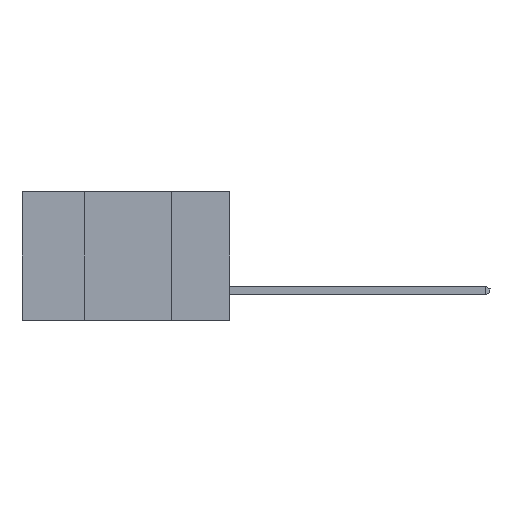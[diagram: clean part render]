
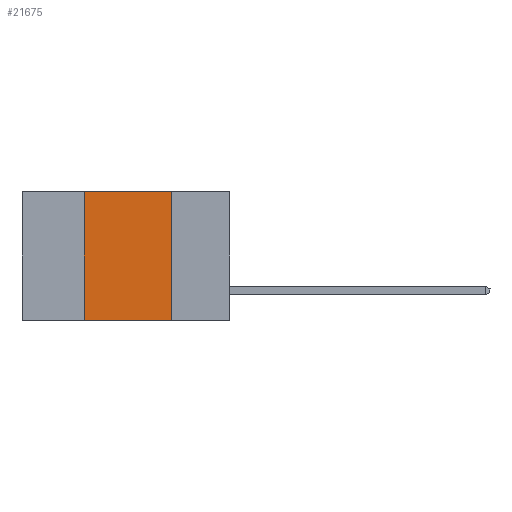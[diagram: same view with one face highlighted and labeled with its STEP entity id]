
A CAD part, left-side view. The second image highlights one B-rep face of the part: STEP entity #21675.
In plain terms, the highlighted planar face has unit normal (-1, 0, 0).
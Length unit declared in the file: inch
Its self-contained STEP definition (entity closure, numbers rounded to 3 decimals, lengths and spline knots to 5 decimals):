
#1277 = CARTESIAN_POINT ( 'NONE',  ( 0., 0.17, -0.37 ) ) ;
#1334 = CARTESIAN_POINT ( 'NONE',  ( 0., 0.6, 0. ) ) ;
#1555 = ORIENTED_EDGE ( 'NONE', *, *, #13676, .F. ) ;
#1757 = VECTOR ( 'NONE', #6043, 39.37008 ) ;
#1799 = DIRECTION ( 'NONE',  ( 1., 0., 0. ) ) ;
#2335 = CARTESIAN_POINT ( 'NONE',  ( 0., 0.42, -0.37 ) ) ;
#2392 = VERTEX_POINT ( 'NONE', #20494 ) ;
#2815 = VERTEX_POINT ( 'NONE', #20209 ) ;
#3241 = EDGE_CURVE ( 'NONE', #14327, #11346, #8127, .T. ) ;
#3512 = DIRECTION ( 'NONE',  ( 0., 0., -1. ) ) ;
#5744 = CARTESIAN_POINT ( 'NONE',  ( 0., 0.17, 0. ) ) ;
#6043 = DIRECTION ( 'NONE',  ( 0., -1., 0. ) ) ;
#7107 = LINE ( 'NONE', #1334, #14543 ) ;
#7436 = CARTESIAN_POINT ( 'NONE',  ( 0., 0.6, 0. ) ) ;
#7623 = CARTESIAN_POINT ( 'NONE',  ( 0., 0.6, -0.37 ) ) ;
#7878 = DIRECTION ( 'NONE',  ( 0., 0., -1. ) ) ;
#8127 = LINE ( 'NONE', #23838, #14890 ) ;
#10889 = ORIENTED_EDGE ( 'NONE', *, *, #11094, .F. ) ;
#11094 = EDGE_CURVE ( 'NONE', #2392, #2815, #18545, .T. ) ;
#11339 = PLANE ( 'NONE',  #21861 ) ;
#11346 = VERTEX_POINT ( 'NONE', #1277 ) ;
#11598 = FACE_OUTER_BOUND ( 'NONE', #17929, .T. ) ;
#12001 = DIRECTION ( 'NONE',  ( 0., 0., 1. ) ) ;
#13260 = VECTOR ( 'NONE', #12001, 39.37008 ) ;
#13676 = EDGE_CURVE ( 'NONE', #2815, #14327, #7107, .T. ) ;
#14327 = VERTEX_POINT ( 'NONE', #5744 ) ;
#14543 = VECTOR ( 'NONE', #22932, 39.37008 ) ;
#14741 = ORIENTED_EDGE ( 'NONE', *, *, #3241, .F. ) ;
#14890 = VECTOR ( 'NONE', #7878, 39.37008 ) ;
#15587 = LINE ( 'NONE', #7623, #1757 ) ;
#17929 = EDGE_LOOP ( 'NONE', ( #14741, #1555, #10889, #21774 ) ) ;
#18545 = LINE ( 'NONE', #2335, #13260 ) ;
#20209 = CARTESIAN_POINT ( 'NONE',  ( 0., 0.42, 0. ) ) ;
#20494 = CARTESIAN_POINT ( 'NONE',  ( 0., 0.42, -0.37 ) ) ;
#21675 = ADVANCED_FACE ( 'NONE', ( #11598 ), #11339, .F. ) ;
#21774 = ORIENTED_EDGE ( 'NONE', *, *, #25368, .T. ) ;
#21861 = AXIS2_PLACEMENT_3D ( 'NONE', #7436, #1799, #3512 ) ;
#22932 = DIRECTION ( 'NONE',  ( 0., -1., 0. ) ) ;
#23838 = CARTESIAN_POINT ( 'NONE',  ( 0., 0.17, -0.37 ) ) ;
#25368 = EDGE_CURVE ( 'NONE', #2392, #11346, #15587, .T. ) ;
